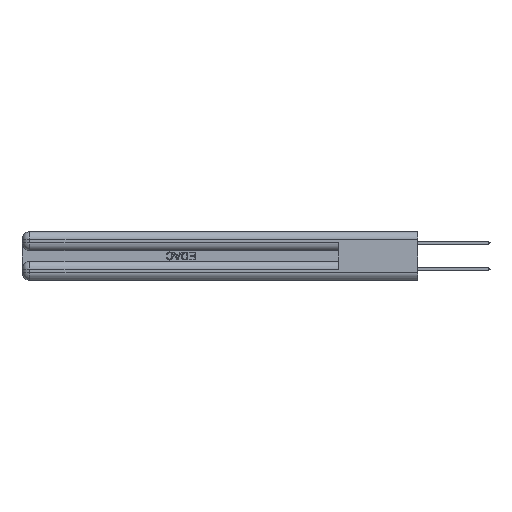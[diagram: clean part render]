
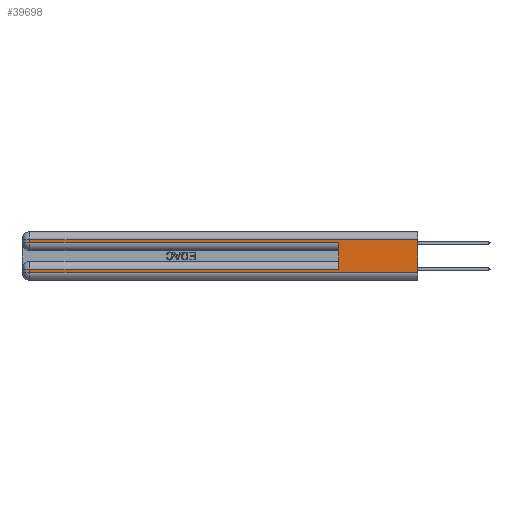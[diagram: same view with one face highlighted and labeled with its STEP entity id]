
A CAD part, left-side view. The second image highlights one B-rep face of the part: STEP entity #39698.
In plain terms, the highlighted planar face has unit normal (-1, 0, 0).
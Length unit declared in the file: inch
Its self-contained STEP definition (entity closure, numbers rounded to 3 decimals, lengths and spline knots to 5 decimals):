
#2332 = DIRECTION ( 'NONE',  ( 0., 0., -1. ) ) ;
#2806 = CARTESIAN_POINT ( 'NONE',  ( 0., 0., 0.37 ) ) ;
#2808 = ORIENTED_EDGE ( 'NONE', *, *, #38632, .T. ) ;
#3073 = FACE_OUTER_BOUND ( 'NONE', #23609, .T. ) ;
#3170 = CARTESIAN_POINT ( 'NONE',  ( 0., 2.94, 0.31 ) ) ;
#3181 = CARTESIAN_POINT ( 'NONE',  ( 0., 0.6, 0.145 ) ) ;
#3253 = CARTESIAN_POINT ( 'NONE',  ( 0., 0., 0.285 ) ) ;
#3281 = VECTOR ( 'NONE', #26552, 39.37008 ) ;
#3997 = DIRECTION ( 'NONE',  ( 1., 0., 0. ) ) ;
#4709 = VECTOR ( 'NONE', #26839, 39.37008 ) ;
#4745 = VERTEX_POINT ( 'NONE', #20541 ) ;
#6543 = LINE ( 'NONE', #18719, #36311 ) ;
#6922 = LINE ( 'NONE', #3253, #25415 ) ;
#8344 = DIRECTION ( 'NONE',  ( 0., 0., -1. ) ) ;
#9177 = EDGE_CURVE ( 'NONE', #29085, #40808, #10832, .T. ) ;
#10832 = LINE ( 'NONE', #25452, #18821 ) ;
#18197 = VERTEX_POINT ( 'NONE', #35362 ) ;
#18719 = CARTESIAN_POINT ( 'NONE',  ( 0., 0., 0.085 ) ) ;
#18821 = VECTOR ( 'NONE', #2332, 39.37008 ) ;
#18962 = EDGE_CURVE ( 'NONE', #4745, #33608, #28211, .T. ) ;
#19423 = CARTESIAN_POINT ( 'NONE',  ( 0., 0., 0.06 ) ) ;
#19667 = VERTEX_POINT ( 'NONE', #27605 ) ;
#20278 = DIRECTION ( 'NONE',  ( 0., 0., -1. ) ) ;
#20449 = CARTESIAN_POINT ( 'NONE',  ( 0., 0., 0.37 ) ) ;
#20541 = CARTESIAN_POINT ( 'NONE',  ( 0., 2.94, 0.085 ) ) ;
#20809 = VECTOR ( 'NONE', #20278, 39.37008 ) ;
#21898 = CARTESIAN_POINT ( 'NONE',  ( 0., 0., 0.31 ) ) ;
#23028 = DIRECTION ( 'NONE',  ( 0., 1., 0. ) ) ;
#23609 = EDGE_LOOP ( 'NONE', ( #42118, #43137, #45821, #31287, #50014, #27684, #45693, #2808 ) ) ;
#24449 = DIRECTION ( 'NONE',  ( 0., -1., 0. ) ) ;
#25415 = VECTOR ( 'NONE', #38706, 39.37008 ) ;
#25452 = CARTESIAN_POINT ( 'NONE',  ( 0., 2.94, 0.37 ) ) ;
#26552 = DIRECTION ( 'NONE',  ( 0., 1., 0. ) ) ;
#26839 = DIRECTION ( 'NONE',  ( 0., 0., 1. ) ) ;
#27605 = CARTESIAN_POINT ( 'NONE',  ( 0., 0., 0.31 ) ) ;
#27684 = ORIENTED_EDGE ( 'NONE', *, *, #32403, .T. ) ;
#27814 = DIRECTION ( 'NONE',  ( 0., 0., -1. ) ) ;
#28211 = LINE ( 'NONE', #32025, #30119 ) ;
#28430 = EDGE_CURVE ( 'NONE', #19667, #29085, #37358, .T. ) ;
#28439 = CARTESIAN_POINT ( 'NONE',  ( 0., 0.6, 0.285 ) ) ;
#29085 = VERTEX_POINT ( 'NONE', #3170 ) ;
#30044 = LINE ( 'NONE', #3181, #4709 ) ;
#30119 = VECTOR ( 'NONE', #8344, 39.37008 ) ;
#31287 = ORIENTED_EDGE ( 'NONE', *, *, #46678, .T. ) ;
#32025 = CARTESIAN_POINT ( 'NONE',  ( 0., 2.94, 0.37 ) ) ;
#32403 = EDGE_CURVE ( 'NONE', #18197, #4745, #6543, .T. ) ;
#33608 = VERTEX_POINT ( 'NONE', #46851 ) ;
#35362 = CARTESIAN_POINT ( 'NONE',  ( 0., 0.6, 0.085 ) ) ;
#36311 = VECTOR ( 'NONE', #23028, 39.37008 ) ;
#36503 = AXIS2_PLACEMENT_3D ( 'NONE', #2806, #3997, #27814 ) ;
#37358 = LINE ( 'NONE', #21898, #3281 ) ;
#38632 = EDGE_CURVE ( 'NONE', #33608, #47193, #50688, .T. ) ;
#38706 = DIRECTION ( 'NONE',  ( 0., -1., 0. ) ) ;
#39698 = ADVANCED_FACE ( 'NONE', ( #3073 ), #46245, .F. ) ;
#40236 = CARTESIAN_POINT ( 'NONE',  ( 0., 0., 0.06 ) ) ;
#40653 = LINE ( 'NONE', #20449, #20809 ) ;
#40808 = VERTEX_POINT ( 'NONE', #41610 ) ;
#40816 = EDGE_CURVE ( 'NONE', #18197, #47453, #30044, .T. ) ;
#41610 = CARTESIAN_POINT ( 'NONE',  ( 0., 2.94, 0.285 ) ) ;
#42118 = ORIENTED_EDGE ( 'NONE', *, *, #49166, .F. ) ;
#43137 = ORIENTED_EDGE ( 'NONE', *, *, #28430, .T. ) ;
#45693 = ORIENTED_EDGE ( 'NONE', *, *, #18962, .T. ) ;
#45821 = ORIENTED_EDGE ( 'NONE', *, *, #9177, .T. ) ;
#46245 = PLANE ( 'NONE',  #36503 ) ;
#46678 = EDGE_CURVE ( 'NONE', #40808, #47453, #6922, .T. ) ;
#46851 = CARTESIAN_POINT ( 'NONE',  ( 0., 2.94, 0.06 ) ) ;
#47193 = VERTEX_POINT ( 'NONE', #19423 ) ;
#47453 = VERTEX_POINT ( 'NONE', #28439 ) ;
#49166 = EDGE_CURVE ( 'NONE', #19667, #47193, #40653, .T. ) ;
#49499 = VECTOR ( 'NONE', #24449, 39.37008 ) ;
#50014 = ORIENTED_EDGE ( 'NONE', *, *, #40816, .F. ) ;
#50688 = LINE ( 'NONE', #40236, #49499 ) ;
